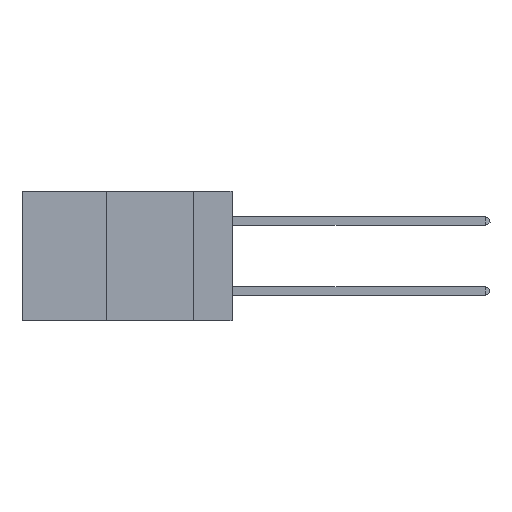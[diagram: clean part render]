
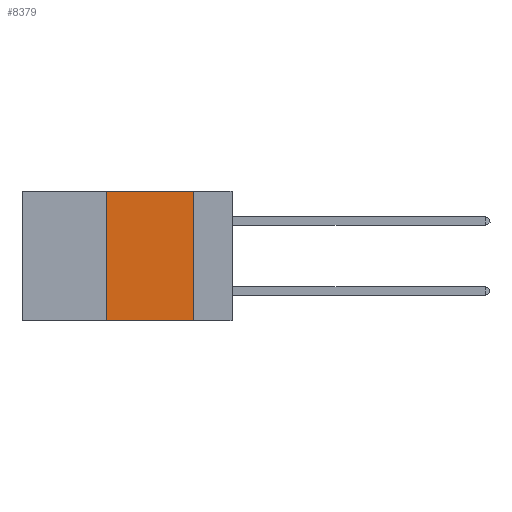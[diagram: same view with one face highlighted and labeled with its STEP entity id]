
A CAD part, left-side view. The second image highlights one B-rep face of the part: STEP entity #8379.
In plain terms, the highlighted planar face has unit normal (-1, 0, 0).
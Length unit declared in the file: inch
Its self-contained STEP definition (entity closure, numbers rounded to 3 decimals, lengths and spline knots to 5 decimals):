
#229 = VERTEX_POINT ( 'NONE', #9522 ) ;
#792 = EDGE_CURVE ( 'NONE', #229, #10075, #10656, .T. ) ;
#1645 = VECTOR ( 'NONE', #8494, 39.37008 ) ;
#2034 = ORIENTED_EDGE ( 'NONE', *, *, #7628, .F. ) ;
#2045 = LINE ( 'NONE', #9159, #7713 ) ;
#2057 = VECTOR ( 'NONE', #11121, 39.37008 ) ;
#2288 = VERTEX_POINT ( 'NONE', #10680 ) ;
#2412 = EDGE_CURVE ( 'NONE', #10075, #11835, #6050, .T. ) ;
#2422 = DIRECTION ( 'NONE',  ( 1., 0., 0. ) ) ;
#2466 = DIRECTION ( 'NONE',  ( 0., -1., 0. ) ) ;
#2469 = CARTESIAN_POINT ( 'NONE',  ( 0., 0.6, 0. ) ) ;
#3549 = DIRECTION ( 'NONE',  ( 0., 0., -1. ) ) ;
#3874 = AXIS2_PLACEMENT_3D ( 'NONE', #2469, #2422, #3549 ) ;
#4337 = CARTESIAN_POINT ( 'NONE',  ( 0., 0.11, 0. ) ) ;
#4512 = PLANE ( 'NONE',  #3874 ) ;
#6050 = LINE ( 'NONE', #9552, #1645 ) ;
#7174 = EDGE_LOOP ( 'NONE', ( #7867, #13290, #2034, #7592 ) ) ;
#7592 = ORIENTED_EDGE ( 'NONE', *, *, #14492, .T. ) ;
#7628 = EDGE_CURVE ( 'NONE', #2288, #229, #10312, .T. ) ;
#7705 = VECTOR ( 'NONE', #8611, 39.37008 ) ;
#7713 = VECTOR ( 'NONE', #2466, 39.37008 ) ;
#7867 = ORIENTED_EDGE ( 'NONE', *, *, #2412, .F. ) ;
#8379 = ADVANCED_FACE ( 'NONE', ( #10811 ), #4512, .F. ) ;
#8494 = DIRECTION ( 'NONE',  ( 0., 0., -1. ) ) ;
#8611 = DIRECTION ( 'NONE',  ( 0., -1., 0. ) ) ;
#9159 = CARTESIAN_POINT ( 'NONE',  ( 0., 0.6, -0.37 ) ) ;
#9522 = CARTESIAN_POINT ( 'NONE',  ( 0., 0.36, 0. ) ) ;
#9552 = CARTESIAN_POINT ( 'NONE',  ( 0., 0.11, 0. ) ) ;
#10075 = VERTEX_POINT ( 'NONE', #4337 ) ;
#10312 = LINE ( 'NONE', #14586, #2057 ) ;
#10656 = LINE ( 'NONE', #13054, #7705 ) ;
#10680 = CARTESIAN_POINT ( 'NONE',  ( 0., 0.36, -0.37 ) ) ;
#10811 = FACE_OUTER_BOUND ( 'NONE', #7174, .T. ) ;
#11121 = DIRECTION ( 'NONE',  ( 0., 0., 1. ) ) ;
#11835 = VERTEX_POINT ( 'NONE', #12312 ) ;
#12312 = CARTESIAN_POINT ( 'NONE',  ( 0., 0.11, -0.37 ) ) ;
#13054 = CARTESIAN_POINT ( 'NONE',  ( 0., 0.6, 0. ) ) ;
#13290 = ORIENTED_EDGE ( 'NONE', *, *, #792, .F. ) ;
#14492 = EDGE_CURVE ( 'NONE', #2288, #11835, #2045, .T. ) ;
#14586 = CARTESIAN_POINT ( 'NONE',  ( 0., 0.36, 0. ) ) ;
